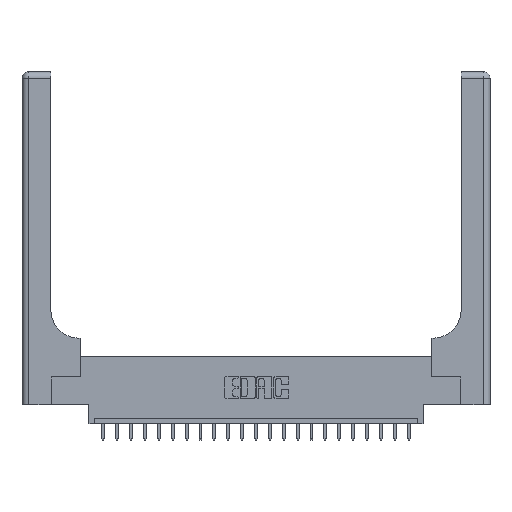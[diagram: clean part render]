
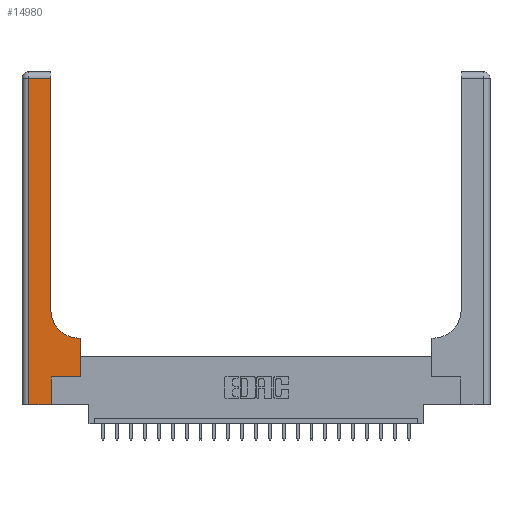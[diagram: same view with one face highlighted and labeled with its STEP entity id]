
A CAD part, top view. The second image highlights one B-rep face of the part: STEP entity #14980.
In plain terms, the highlighted planar face has unit normal (0, 0, 1).
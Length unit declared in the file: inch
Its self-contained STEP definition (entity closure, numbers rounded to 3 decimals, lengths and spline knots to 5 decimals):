
#103 = CARTESIAN_POINT ( 'NONE',  ( 0.06, 0., 0.37 ) ) ;
#748 = CARTESIAN_POINT ( 'NONE',  ( 0.265, 0.25, 0.37 ) ) ;
#777 = CARTESIAN_POINT ( 'NONE',  ( 0.26, 2.94, 0.37 ) ) ;
#944 = EDGE_CURVE ( 'NONE', #11807, #6635, #1575, .T. ) ;
#1237 = CARTESIAN_POINT ( 'NONE',  ( 0.26, 0.6, 0.37 ) ) ;
#1540 = CARTESIAN_POINT ( 'NONE',  ( 0.528, 0.6, 0.37 ) ) ;
#1575 = LINE ( 'NONE', #1766, #9119 ) ;
#1766 = CARTESIAN_POINT ( 'NONE',  ( 0., 0., 0.37 ) ) ;
#1832 = AXIS2_PLACEMENT_3D ( 'NONE', #8618, #7030, #17091 ) ;
#1908 = CARTESIAN_POINT ( 'NONE',  ( 0., 2.94, 0.37 ) ) ;
#2197 = ORIENTED_EDGE ( 'NONE', *, *, #11226, .T. ) ;
#2278 = LINE ( 'NONE', #16674, #8743 ) ;
#2849 = ORIENTED_EDGE ( 'NONE', *, *, #7215, .T. ) ;
#3530 = VERTEX_POINT ( 'NONE', #11932 ) ;
#3814 = CIRCLE ( 'NONE', #1832, 0.25 ) ;
#4110 = CARTESIAN_POINT ( 'NONE',  ( 0.51, 0.6, 0.37 ) ) ;
#4186 = DIRECTION ( 'NONE',  ( -1., 0., 0. ) ) ;
#4537 = VECTOR ( 'NONE', #16670, 39.37008 ) ;
#4824 = VERTEX_POINT ( 'NONE', #5923 ) ;
#4965 = CARTESIAN_POINT ( 'NONE',  ( 0.265, 0., 0.37 ) ) ;
#5787 = ORIENTED_EDGE ( 'NONE', *, *, #20203, .T. ) ;
#5804 = DIRECTION ( 'NONE',  ( 0., 1., 0. ) ) ;
#5837 = LINE ( 'NONE', #13190, #4537 ) ;
#5894 = DIRECTION ( 'NONE',  ( 0., 0., -1. ) ) ;
#5923 = CARTESIAN_POINT ( 'NONE',  ( 0.265, 0.25, 0.37 ) ) ;
#6635 = VERTEX_POINT ( 'NONE', #4965 ) ;
#6687 = EDGE_LOOP ( 'NONE', ( #5787, #2197, #9042, #13495, #14206, #2849, #13845, #17281, #8817 ) ) ;
#7030 = DIRECTION ( 'NONE',  ( 0., 0., -1. ) ) ;
#7215 = EDGE_CURVE ( 'NONE', #4824, #21633, #20613, .T. ) ;
#7294 = FACE_OUTER_BOUND ( 'NONE', #6687, .T. ) ;
#7916 = DIRECTION ( 'NONE',  ( -1., 0., 0. ) ) ;
#8618 = CARTESIAN_POINT ( 'NONE',  ( 0.51, 0.85, 0.37 ) ) ;
#8743 = VECTOR ( 'NONE', #18378, 39.37008 ) ;
#8817 = ORIENTED_EDGE ( 'NONE', *, *, #14184, .T. ) ;
#9042 = ORIENTED_EDGE ( 'NONE', *, *, #15427, .T. ) ;
#9119 = VECTOR ( 'NONE', #15694, 39.37008 ) ;
#9244 = CARTESIAN_POINT ( 'NONE',  ( 0.265, 0., 0.37 ) ) ;
#9392 = CARTESIAN_POINT ( 'NONE',  ( 0., 3., 0.37 ) ) ;
#9905 = AXIS2_PLACEMENT_3D ( 'NONE', #9392, #5894, #4186 ) ;
#10156 = LINE ( 'NONE', #1237, #12303 ) ;
#10189 = DIRECTION ( 'NONE',  ( 1., 0., 0. ) ) ;
#10610 = EDGE_CURVE ( 'NONE', #21633, #20282, #2278, .T. ) ;
#10616 = VECTOR ( 'NONE', #18934, 39.37008 ) ;
#11040 = VECTOR ( 'NONE', #15653, 39.37008 ) ;
#11226 = EDGE_CURVE ( 'NONE', #14356, #11916, #20742, .T. ) ;
#11807 = VERTEX_POINT ( 'NONE', #103 ) ;
#11916 = VERTEX_POINT ( 'NONE', #12186 ) ;
#11932 = CARTESIAN_POINT ( 'NONE',  ( 0.26, 0.85, 0.37 ) ) ;
#12186 = CARTESIAN_POINT ( 'NONE',  ( 0.06, 2.94, 0.37 ) ) ;
#12303 = VECTOR ( 'NONE', #7916, 39.37008 ) ;
#12314 = EDGE_CURVE ( 'NONE', #6635, #4824, #17843, .T. ) ;
#13190 = CARTESIAN_POINT ( 'NONE',  ( 0.26, 3., 0.37 ) ) ;
#13495 = ORIENTED_EDGE ( 'NONE', *, *, #944, .T. ) ;
#13845 = ORIENTED_EDGE ( 'NONE', *, *, #10610, .T. ) ;
#14086 = CARTESIAN_POINT ( 'NONE',  ( 0.528, 0.25, 0.37 ) ) ;
#14184 = EDGE_CURVE ( 'NONE', #20139, #3530, #3814, .T. ) ;
#14206 = ORIENTED_EDGE ( 'NONE', *, *, #12314, .T. ) ;
#14356 = VERTEX_POINT ( 'NONE', #777 ) ;
#14980 = ADVANCED_FACE ( 'NONE', ( #7294 ), #17864, .F. ) ;
#15167 = VECTOR ( 'NONE', #5804, 39.37008 ) ;
#15427 = EDGE_CURVE ( 'NONE', #11916, #11807, #15829, .T. ) ;
#15653 = DIRECTION ( 'NONE',  ( 0., -1., 0. ) ) ;
#15694 = DIRECTION ( 'NONE',  ( 1., 0., 0. ) ) ;
#15829 = LINE ( 'NONE', #20714, #11040 ) ;
#16670 = DIRECTION ( 'NONE',  ( 0., 1., 0. ) ) ;
#16674 = CARTESIAN_POINT ( 'NONE',  ( 0.528, 0.25, 0.37 ) ) ;
#16849 = EDGE_CURVE ( 'NONE', #20282, #20139, #10156, .T. ) ;
#17091 = DIRECTION ( 'NONE',  ( 1., 0., 0. ) ) ;
#17281 = ORIENTED_EDGE ( 'NONE', *, *, #16849, .T. ) ;
#17843 = LINE ( 'NONE', #9244, #15167 ) ;
#17864 = PLANE ( 'NONE',  #9905 ) ;
#18378 = DIRECTION ( 'NONE',  ( 0., 1., 0. ) ) ;
#18934 = DIRECTION ( 'NONE',  ( -1., 0., 0. ) ) ;
#18993 = VECTOR ( 'NONE', #10189, 39.37008 ) ;
#20139 = VERTEX_POINT ( 'NONE', #4110 ) ;
#20203 = EDGE_CURVE ( 'NONE', #3530, #14356, #5837, .T. ) ;
#20282 = VERTEX_POINT ( 'NONE', #1540 ) ;
#20613 = LINE ( 'NONE', #748, #18993 ) ;
#20714 = CARTESIAN_POINT ( 'NONE',  ( 0.06, 3., 0.37 ) ) ;
#20742 = LINE ( 'NONE', #1908, #10616 ) ;
#21633 = VERTEX_POINT ( 'NONE', #14086 ) ;
